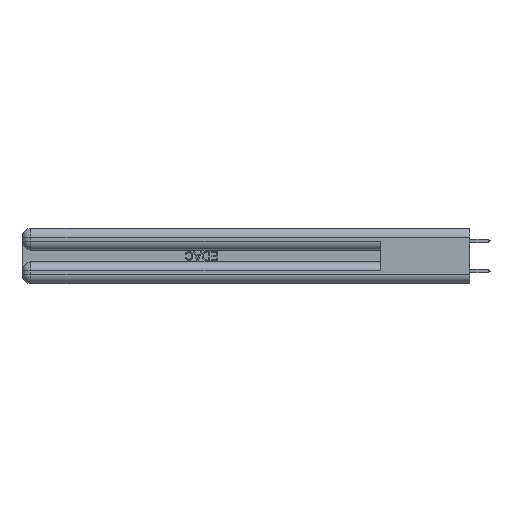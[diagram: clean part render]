
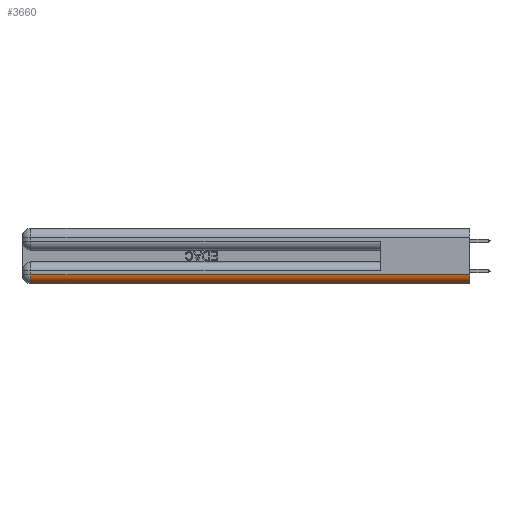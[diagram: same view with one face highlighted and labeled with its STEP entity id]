
A CAD part, left-side view. The second image highlights one B-rep face of the part: STEP entity #3660.
In plain terms, the highlighted cylindrical face has radius 1.524 mm (diameter 3.048 mm), a partial arc.
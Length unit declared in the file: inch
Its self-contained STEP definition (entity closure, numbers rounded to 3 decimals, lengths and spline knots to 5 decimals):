
#801 = DIRECTION ( 'NONE',  ( 0., -1., 0. ) ) ;
#2106 = CYLINDRICAL_SURFACE ( 'NONE', #3406, 0.06 ) ;
#3122 = FACE_OUTER_BOUND ( 'NONE', #30488, .T. ) ;
#3406 = AXIS2_PLACEMENT_3D ( 'NONE', #40586, #24155, #11024 ) ;
#3660 = ADVANCED_FACE ( 'NONE', ( #3122 ), #2106, .T. ) ;
#4493 = VERTEX_POINT ( 'NONE', #18475 ) ;
#5451 = ORIENTED_EDGE ( 'NONE', *, *, #24454, .F. ) ;
#6365 = VECTOR ( 'NONE', #8855, 39.37008 ) ;
#6461 = DIRECTION ( 'NONE',  ( 0., 1., 0. ) ) ;
#8855 = DIRECTION ( 'NONE',  ( 0., -1., 0. ) ) ;
#11024 = DIRECTION ( 'NONE',  ( 0., 0., 1. ) ) ;
#11170 = AXIS2_PLACEMENT_3D ( 'NONE', #26247, #6461, #29559 ) ;
#13146 = CIRCLE ( 'NONE', #20961, 0.06 ) ;
#17412 = EDGE_CURVE ( 'NONE', #4493, #31384, #13146, .T. ) ;
#17812 = EDGE_CURVE ( 'NONE', #40213, #4493, #33768, .T. ) ;
#18475 = CARTESIAN_POINT ( 'NONE',  ( 0., 0., 0.06 ) ) ;
#19378 = ORIENTED_EDGE ( 'NONE', *, *, #17412, .F. ) ;
#20572 = CARTESIAN_POINT ( 'NONE',  ( 0.06, 0., 0.06 ) ) ;
#20732 = CARTESIAN_POINT ( 'NONE',  ( 0.06, 3., 0. ) ) ;
#20825 = VECTOR ( 'NONE', #21479, 39.37008 ) ;
#20961 = AXIS2_PLACEMENT_3D ( 'NONE', #20572, #801, #23909 ) ;
#21479 = DIRECTION ( 'NONE',  ( 0., 1., 0. ) ) ;
#22225 = CARTESIAN_POINT ( 'NONE',  ( 0.06, 2.94, 0. ) ) ;
#23909 = DIRECTION ( 'NONE',  ( 0., 0., 1. ) ) ;
#24155 = DIRECTION ( 'NONE',  ( 0., 1., 0. ) ) ;
#24454 = EDGE_CURVE ( 'NONE', #34807, #40213, #39601, .T. ) ;
#25110 = ORIENTED_EDGE ( 'NONE', *, *, #26697, .F. ) ;
#26247 = CARTESIAN_POINT ( 'NONE',  ( 0.06, 2.94, 0.06 ) ) ;
#26697 = EDGE_CURVE ( 'NONE', #31384, #34807, #30646, .T. ) ;
#28623 = CARTESIAN_POINT ( 'NONE',  ( 0., 0., 0.06 ) ) ;
#29559 = DIRECTION ( 'NONE',  ( 0., 0., 1. ) ) ;
#30488 = EDGE_LOOP ( 'NONE', ( #19378, #34390, #5451, #25110 ) ) ;
#30646 = LINE ( 'NONE', #20732, #20825 ) ;
#31384 = VERTEX_POINT ( 'NONE', #36735 ) ;
#33768 = LINE ( 'NONE', #28623, #6365 ) ;
#34390 = ORIENTED_EDGE ( 'NONE', *, *, #17812, .F. ) ;
#34807 = VERTEX_POINT ( 'NONE', #22225 ) ;
#36735 = CARTESIAN_POINT ( 'NONE',  ( 0.06, 0., 0. ) ) ;
#39252 = CARTESIAN_POINT ( 'NONE',  ( 0., 2.94, 0.06 ) ) ;
#39601 = CIRCLE ( 'NONE', #11170, 0.06 ) ;
#40213 = VERTEX_POINT ( 'NONE', #39252 ) ;
#40586 = CARTESIAN_POINT ( 'NONE',  ( 0.06, 0., 0.06 ) ) ;
